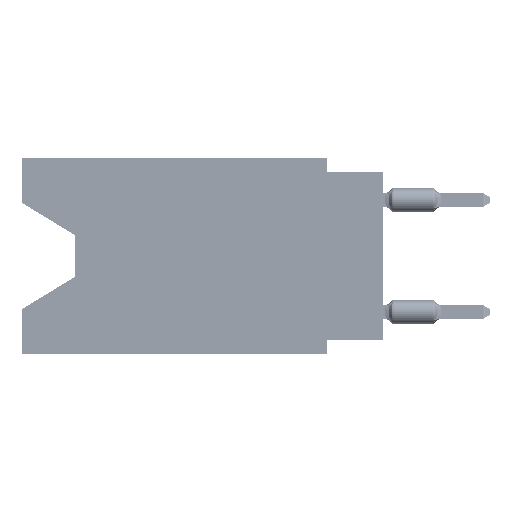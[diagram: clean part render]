
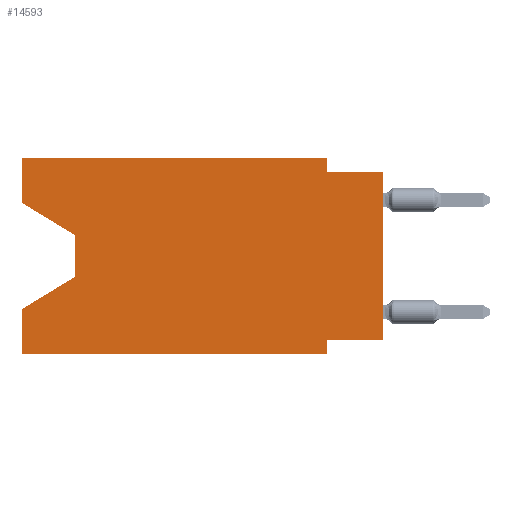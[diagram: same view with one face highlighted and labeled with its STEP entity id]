
A CAD part, left-side view. The second image highlights one B-rep face of the part: STEP entity #14593.
In plain terms, the highlighted planar face has unit normal (-1, 0, 0).
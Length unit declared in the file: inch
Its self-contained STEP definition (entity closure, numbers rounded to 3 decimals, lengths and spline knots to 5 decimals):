
#340 = CARTESIAN_POINT ( 'NONE',  ( 0., 0.55, -0.212 ) ) ;
#1201 = LINE ( 'NONE', #54048, #71684 ) ;
#1372 = CARTESIAN_POINT ( 'NONE',  ( 0., 0.1, -0.35 ) ) ;
#1382 = CARTESIAN_POINT ( 'NONE',  ( 0., 0., -0.025 ) ) ;
#2217 = VERTEX_POINT ( 'NONE', #82441 ) ;
#2853 = DIRECTION ( 'NONE',  ( 0., -0.855, -0.519 ) ) ;
#3174 = CARTESIAN_POINT ( 'NONE',  ( 0., 0.645, 0. ) ) ;
#3743 = DIRECTION ( 'NONE',  ( 0., 0.855, -0.519 ) ) ;
#3819 = PLANE ( 'NONE',  #43358 ) ;
#4194 = DIRECTION ( 'NONE',  ( 0., 0., 1. ) ) ;
#5318 = CARTESIAN_POINT ( 'NONE',  ( 0., 0.645, -0.26975 ) ) ;
#6408 = CARTESIAN_POINT ( 'NONE',  ( 0., 0., -0.325 ) ) ;
#6723 = EDGE_CURVE ( 'NONE', #86753, #18524, #63971, .T. ) ;
#7309 = EDGE_CURVE ( 'NONE', #75259, #86173, #1201, .T. ) ;
#10129 = VERTEX_POINT ( 'NONE', #1382 ) ;
#10578 = VECTOR ( 'NONE', #20804, 39.37008 ) ;
#12226 = CARTESIAN_POINT ( 'NONE',  ( 0., 0.645, 0. ) ) ;
#12656 = DIRECTION ( 'NONE',  ( 0., 1., 0. ) ) ;
#13405 = EDGE_CURVE ( 'NONE', #36931, #2217, #61417, .T. ) ;
#14593 = ADVANCED_FACE ( 'NONE', ( #17555 ), #3819, .F. ) ;
#16480 = VECTOR ( 'NONE', #57320, 39.37008 ) ;
#16732 = CARTESIAN_POINT ( 'NONE',  ( 0., 0.645, 0. ) ) ;
#17157 = LINE ( 'NONE', #16732, #74731 ) ;
#17555 = FACE_OUTER_BOUND ( 'NONE', #47297, .T. ) ;
#17724 = ORIENTED_EDGE ( 'NONE', *, *, #62055, .T. ) ;
#18176 = EDGE_CURVE ( 'NONE', #2217, #87524, #54212, .T. ) ;
#18524 = VERTEX_POINT ( 'NONE', #5318 ) ;
#20690 = VECTOR ( 'NONE', #2853, 39.37008 ) ;
#20804 = DIRECTION ( 'NONE',  ( 0., -1., 0. ) ) ;
#21201 = ORIENTED_EDGE ( 'NONE', *, *, #6723, .F. ) ;
#23665 = ORIENTED_EDGE ( 'NONE', *, *, #32829, .F. ) ;
#24524 = ORIENTED_EDGE ( 'NONE', *, *, #60468, .T. ) ;
#24654 = DIRECTION ( 'NONE',  ( 0., -1., 0. ) ) ;
#26371 = ORIENTED_EDGE ( 'NONE', *, *, #18176, .F. ) ;
#28843 = LINE ( 'NONE', #55913, #34200 ) ;
#30070 = LINE ( 'NONE', #35847, #79387 ) ;
#31981 = VECTOR ( 'NONE', #3743, 39.37008 ) ;
#32829 = EDGE_CURVE ( 'NONE', #86173, #10129, #70857, .T. ) ;
#34200 = VECTOR ( 'NONE', #82990, 39.37008 ) ;
#35817 = CARTESIAN_POINT ( 'NONE',  ( 0., 0.645, -0.08025 ) ) ;
#35847 = CARTESIAN_POINT ( 'NONE',  ( 0., 0.645, 0. ) ) ;
#36843 = VERTEX_POINT ( 'NONE', #37318 ) ;
#36931 = VERTEX_POINT ( 'NONE', #76409 ) ;
#37318 = CARTESIAN_POINT ( 'NONE',  ( 0., 0.55, -0.138 ) ) ;
#37923 = LINE ( 'NONE', #64979, #52920 ) ;
#37988 = CARTESIAN_POINT ( 'NONE',  ( 0., 0., -0.025 ) ) ;
#40811 = ORIENTED_EDGE ( 'NONE', *, *, #13405, .F. ) ;
#41227 = LINE ( 'NONE', #82482, #10578 ) ;
#41522 = CARTESIAN_POINT ( 'NONE',  ( 0., 0.1, 0. ) ) ;
#41623 = VERTEX_POINT ( 'NONE', #35817 ) ;
#41705 = VECTOR ( 'NONE', #24654, 39.37008 ) ;
#41779 = DIRECTION ( 'NONE',  ( 0., 0., -1. ) ) ;
#42933 = DIRECTION ( 'NONE',  ( 0., 0., 1. ) ) ;
#43300 = ORIENTED_EDGE ( 'NONE', *, *, #75454, .T. ) ;
#43358 = AXIS2_PLACEMENT_3D ( 'NONE', #12226, #45509, #65884 ) ;
#43838 = DIRECTION ( 'NONE',  ( 0., -1., 0. ) ) ;
#45509 = DIRECTION ( 'NONE',  ( 1., 0., 0. ) ) ;
#46024 = ORIENTED_EDGE ( 'NONE', *, *, #85135, .T. ) ;
#47297 = EDGE_LOOP ( 'NONE', ( #17724, #46024, #62143, #21201, #24524, #26371, #40811, #43300, #23665, #69834, #78966, #85527 ) ) ;
#48294 = CARTESIAN_POINT ( 'NONE',  ( 0., 0.645, -0.35 ) ) ;
#50454 = VERTEX_POINT ( 'NONE', #58182 ) ;
#52195 = EDGE_CURVE ( 'NONE', #50454, #18524, #61160, .T. ) ;
#52333 = VECTOR ( 'NONE', #12656, 39.37008 ) ;
#52920 = VECTOR ( 'NONE', #4194, 39.37008 ) ;
#53463 = VERTEX_POINT ( 'NONE', #72551 ) ;
#54048 = CARTESIAN_POINT ( 'NONE',  ( 0., 0.1, 0. ) ) ;
#54212 = LINE ( 'NONE', #1372, #79017 ) ;
#55052 = CARTESIAN_POINT ( 'NONE',  ( 0., 0.1, -0.025 ) ) ;
#55913 = CARTESIAN_POINT ( 'NONE',  ( 0., 0.55, -0.138 ) ) ;
#56578 = LINE ( 'NONE', #77002, #20690 ) ;
#57320 = DIRECTION ( 'NONE',  ( 0., 0., 1. ) ) ;
#58182 = CARTESIAN_POINT ( 'NONE',  ( 0., 0.55, -0.212 ) ) ;
#60468 = EDGE_CURVE ( 'NONE', #86753, #87524, #41227, .T. ) ;
#61160 = LINE ( 'NONE', #340, #31981 ) ;
#61417 = LINE ( 'NONE', #6408, #52333 ) ;
#62055 = EDGE_CURVE ( 'NONE', #41623, #36843, #56578, .T. ) ;
#62143 = ORIENTED_EDGE ( 'NONE', *, *, #52195, .T. ) ;
#63915 = CARTESIAN_POINT ( 'NONE',  ( 0., 0.1, -0.35 ) ) ;
#63971 = LINE ( 'NONE', #3174, #16480 ) ;
#64979 = CARTESIAN_POINT ( 'NONE',  ( 0., 0., 0. ) ) ;
#65056 = EDGE_CURVE ( 'NONE', #41623, #53463, #17157, .T. ) ;
#65884 = DIRECTION ( 'NONE',  ( 0., 0., -1. ) ) ;
#69834 = ORIENTED_EDGE ( 'NONE', *, *, #7309, .F. ) ;
#70857 = LINE ( 'NONE', #37988, #41705 ) ;
#71684 = VECTOR ( 'NONE', #82433, 39.37008 ) ;
#72551 = CARTESIAN_POINT ( 'NONE',  ( 0., 0.645, 0. ) ) ;
#74731 = VECTOR ( 'NONE', #42933, 39.37008 ) ;
#75259 = VERTEX_POINT ( 'NONE', #41522 ) ;
#75454 = EDGE_CURVE ( 'NONE', #36931, #10129, #37923, .T. ) ;
#76409 = CARTESIAN_POINT ( 'NONE',  ( 0., 0., -0.325 ) ) ;
#77002 = CARTESIAN_POINT ( 'NONE',  ( 0., 0.645, -0.08025 ) ) ;
#78966 = ORIENTED_EDGE ( 'NONE', *, *, #83632, .F. ) ;
#79017 = VECTOR ( 'NONE', #41779, 39.37008 ) ;
#79387 = VECTOR ( 'NONE', #43838, 39.37008 ) ;
#82433 = DIRECTION ( 'NONE',  ( 0., 0., -1. ) ) ;
#82441 = CARTESIAN_POINT ( 'NONE',  ( 0., 0.1, -0.325 ) ) ;
#82482 = CARTESIAN_POINT ( 'NONE',  ( 0., 0.645, -0.35 ) ) ;
#82990 = DIRECTION ( 'NONE',  ( 0., 0., -1. ) ) ;
#83632 = EDGE_CURVE ( 'NONE', #53463, #75259, #30070, .T. ) ;
#85135 = EDGE_CURVE ( 'NONE', #36843, #50454, #28843, .T. ) ;
#85527 = ORIENTED_EDGE ( 'NONE', *, *, #65056, .F. ) ;
#86173 = VERTEX_POINT ( 'NONE', #55052 ) ;
#86753 = VERTEX_POINT ( 'NONE', #48294 ) ;
#87524 = VERTEX_POINT ( 'NONE', #63915 ) ;
